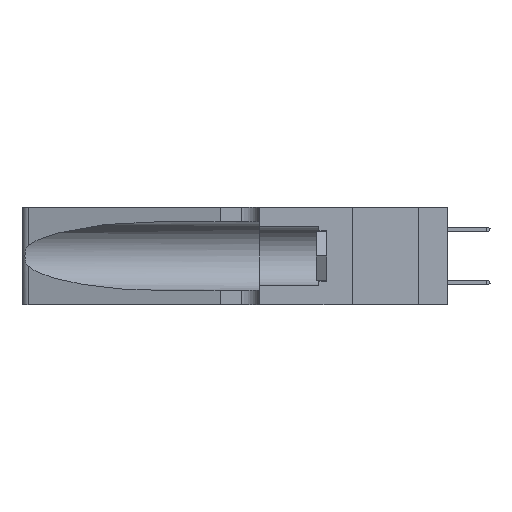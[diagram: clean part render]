
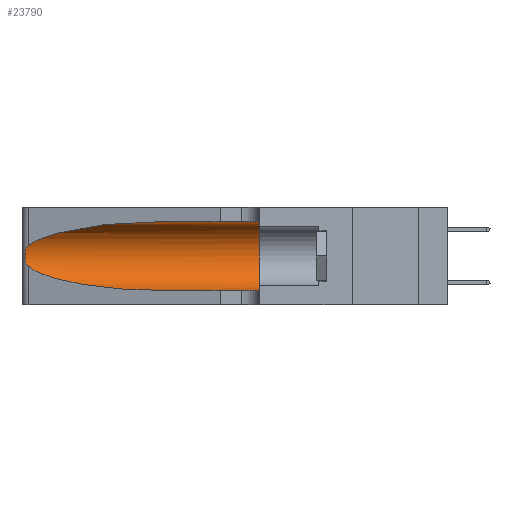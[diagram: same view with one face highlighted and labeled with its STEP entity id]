
A CAD part, left-side view. The second image highlights one B-rep face of the part: STEP entity #23790.
In plain terms, the highlighted cylindrical face has radius 3.308 mm (diameter 6.617 mm), a partial arc.
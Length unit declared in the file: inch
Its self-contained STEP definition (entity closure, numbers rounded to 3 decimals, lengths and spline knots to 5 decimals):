
#667 = CARTESIAN_POINT ( 'NONE',  ( 0.25487, 1.22718, 0.14631 ) ) ;
#777 = CARTESIAN_POINT ( 'NONE',  ( 0.2373, 1.15595, 0.28018 ) ) ;
#1687 = CARTESIAN_POINT ( 'NONE',  ( 0.25789, 1.23486, 0.15765 ) ) ;
#2864 = EDGE_CURVE ( 'NONE', #35756, #28980, #35364, .T. ) ;
#4648 = CARTESIAN_POINT ( 'NONE',  ( 0.25487, 1.22718, 0.22369 ) ) ;
#4787 = CARTESIAN_POINT ( 'NONE',  ( 0.25555, 1.22993, 0.14849 ) ) ;
#5014 = DIRECTION ( 'NONE',  ( 0., 0., -1. ) ) ;
#5415 = CARTESIAN_POINT ( 'NONE',  ( 0.1305, 0.35, 0.05475 ) ) ;
#6303 = CIRCLE ( 'NONE', #9525, 0.13025 ) ;
#6902 = VERTEX_POINT ( 'NONE', #18664 ) ;
#9080 = AXIS2_PLACEMENT_3D ( 'NONE', #26404, #11427, #5014 ) ;
#9193 = CARTESIAN_POINT ( 'NONE',  ( 0.1305, 0.35, 0.185 ) ) ;
#9469 = CARTESIAN_POINT ( 'NONE',  ( 0.1305, 1.61858, 0.31525 ) ) ;
#9511 = DIRECTION ( 'NONE',  ( 0., -1., 0. ) ) ;
#9525 = AXIS2_PLACEMENT_3D ( 'NONE', #9193, #30255, #12209 ) ;
#9560 = CARTESIAN_POINT ( 'NONE',  ( 0.2373, 1.15595, 0.08982 ) ) ;
#9693 = CARTESIAN_POINT ( 'NONE',  ( 0.18966, 0.96281, 0.05475 ) ) ;
#10811 = CARTESIAN_POINT ( 'NONE',  ( 0.25787, 1.23484, 0.2124 ) ) ;
#10847 = CARTESIAN_POINT ( 'NONE',  ( 0.1305, 0.72297, 0.05475 ) ) ;
#11209 = ORIENTED_EDGE ( 'NONE', *, *, #16632, .T. ) ;
#11427 = DIRECTION ( 'NONE',  ( 0., -1., 0. ) ) ;
#11536 = VECTOR ( 'NONE', #36617, 39.37008 ) ;
#12209 = DIRECTION ( 'NONE',  ( 0., 0., 1. ) ) ;
#12703 = CARTESIAN_POINT ( 'NONE',  ( 0.1305, 0.72297, 0.05475 ) ) ;
#12916 = VERTEX_POINT ( 'NONE', #26895 ) ;
#13120 =( BOUNDED_CURVE ( )  B_SPLINE_CURVE ( 3, ( #37066, #19044, #777, #22024 ),
 .UNSPECIFIED., .F., .F. ) 
 B_SPLINE_CURVE_WITH_KNOTS ( ( 4, 4 ),
 ( 1.5708, 2.84003 ),
 .UNSPECIFIED. ) 
 CURVE ( )  GEOMETRIC_REPRESENTATION_ITEM ( )  RATIONAL_B_SPLINE_CURVE ( ( 1., 0.87, 0.87, 1. ) ) 
 REPRESENTATION_ITEM ( '' )  );
#13832 = CARTESIAN_POINT ( 'NONE',  ( 0.26018, 1.23835, 0.19895 ) ) ;
#15574 = CARTESIAN_POINT ( 'NONE',  ( 0.1305, 1.61858, 0.05475 ) ) ;
#15626 = VECTOR ( 'NONE', #9511, 39.37008 ) ;
#16562 = LINE ( 'NONE', #15574, #15626 ) ;
#16632 = EDGE_CURVE ( 'NONE', #12916, #35756, #31241, .T. ) ;
#16866 = CARTESIAN_POINT ( 'NONE',  ( 0.26075, 1.23896, 0.178 ) ) ;
#17842 = ORIENTED_EDGE ( 'NONE', *, *, #39073, .F. ) ;
#18157 = ORIENTED_EDGE ( 'NONE', *, *, #27056, .T. ) ;
#18664 = CARTESIAN_POINT ( 'NONE',  ( 0.1305, 0.35, 0.31525 ) ) ;
#19044 = CARTESIAN_POINT ( 'NONE',  ( 0.18966, 0.96281, 0.31525 ) ) ;
#19919 = CARTESIAN_POINT ( 'NONE',  ( 0.25856, 1.23593, 0.16098 ) ) ;
#22024 = CARTESIAN_POINT ( 'NONE',  ( 0.25487, 1.22718, 0.22369 ) ) ;
#22884 = CARTESIAN_POINT ( 'NONE',  ( 0.25639, 1.23186, 0.15144 ) ) ;
#23790 = ADVANCED_FACE ( 'NONE', ( #28997 ), #36097, .F. ) ;
#24647 = CARTESIAN_POINT ( 'NONE',  ( 0.25487, 1.22718, 0.14631 ) ) ;
#25776 = CARTESIAN_POINT ( 'NONE',  ( 0.25555, 1.22994, 0.2215 ) ) ;
#25911 = CARTESIAN_POINT ( 'NONE',  ( 0.25487, 1.22718, 0.14631 ) ) ;
#26050 = ORIENTED_EDGE ( 'NONE', *, *, #36386, .T. ) ;
#26404 = CARTESIAN_POINT ( 'NONE',  ( 0.1305, 1.61858, 0.185 ) ) ;
#26598 = ORIENTED_EDGE ( 'NONE', *, *, #28123, .F. ) ;
#26895 = CARTESIAN_POINT ( 'NONE',  ( 0.25487, 1.22718, 0.22369 ) ) ;
#27056 = EDGE_CURVE ( 'NONE', #28980, #31856, #16562, .T. ) ;
#28123 = EDGE_CURVE ( 'NONE', #31730, #6902, #35599, .T. ) ;
#28424 = CARTESIAN_POINT ( 'NONE',  ( 0.1305, 0.72297, 0.31525 ) ) ;
#28851 = CARTESIAN_POINT ( 'NONE',  ( 0.25639, 1.23184, 0.21858 ) ) ;
#28980 = VERTEX_POINT ( 'NONE', #10847 ) ;
#28997 = FACE_OUTER_BOUND ( 'NONE', #35876, .T. ) ;
#30255 = DIRECTION ( 'NONE',  ( 0., 1., 0. ) ) ;
#31241 = B_SPLINE_CURVE_WITH_KNOTS ( 'NONE', 3,
 ( #4648, #25776, #28851, #10811, #31900, #13832, #34944, #16866, #37921, #19919, #1687, #22884, #4787, #25911 ),
 .UNSPECIFIED., .F., .F.,
 ( 4, 2, 2, 2, 2, 2, 4 ),
 ( 0., 0.00027, 0.00053, 0.00107, 0.0016, 0.00187, 0.00214 ),
 .UNSPECIFIED. ) ;
#31730 = VERTEX_POINT ( 'NONE', #28424 ) ;
#31856 = VERTEX_POINT ( 'NONE', #5415 ) ;
#31900 = CARTESIAN_POINT ( 'NONE',  ( 0.25854, 1.2359, 0.20912 ) ) ;
#34944 = CARTESIAN_POINT ( 'NONE',  ( 0.26075, 1.23896, 0.19203 ) ) ;
#35364 =( BOUNDED_CURVE ( )  B_SPLINE_CURVE ( 3, ( #24647, #9560, #9693, #12703 ),
 .UNSPECIFIED., .F., .F. ) 
 B_SPLINE_CURVE_WITH_KNOTS ( ( 4, 4 ),
 ( 3.44316, 4.71239 ),
 .UNSPECIFIED. ) 
 CURVE ( )  GEOMETRIC_REPRESENTATION_ITEM ( )  RATIONAL_B_SPLINE_CURVE ( ( 1., 0.87, 0.87, 1. ) ) 
 REPRESENTATION_ITEM ( '' )  );
#35599 = LINE ( 'NONE', #9469, #11536 ) ;
#35756 = VERTEX_POINT ( 'NONE', #667 ) ;
#35876 = EDGE_LOOP ( 'NONE', ( #26050, #11209, #37322, #18157, #17842, #26598 ) ) ;
#36097 = CYLINDRICAL_SURFACE ( 'NONE', #9080, 0.13025 ) ;
#36386 = EDGE_CURVE ( 'NONE', #31730, #12916, #13120, .T. ) ;
#36617 = DIRECTION ( 'NONE',  ( 0., -1., 0. ) ) ;
#37066 = CARTESIAN_POINT ( 'NONE',  ( 0.1305, 0.72297, 0.31525 ) ) ;
#37322 = ORIENTED_EDGE ( 'NONE', *, *, #2864, .T. ) ;
#37921 = CARTESIAN_POINT ( 'NONE',  ( 0.26017, 1.23833, 0.17102 ) ) ;
#39073 = EDGE_CURVE ( 'NONE', #6902, #31856, #6303, .T. ) ;
